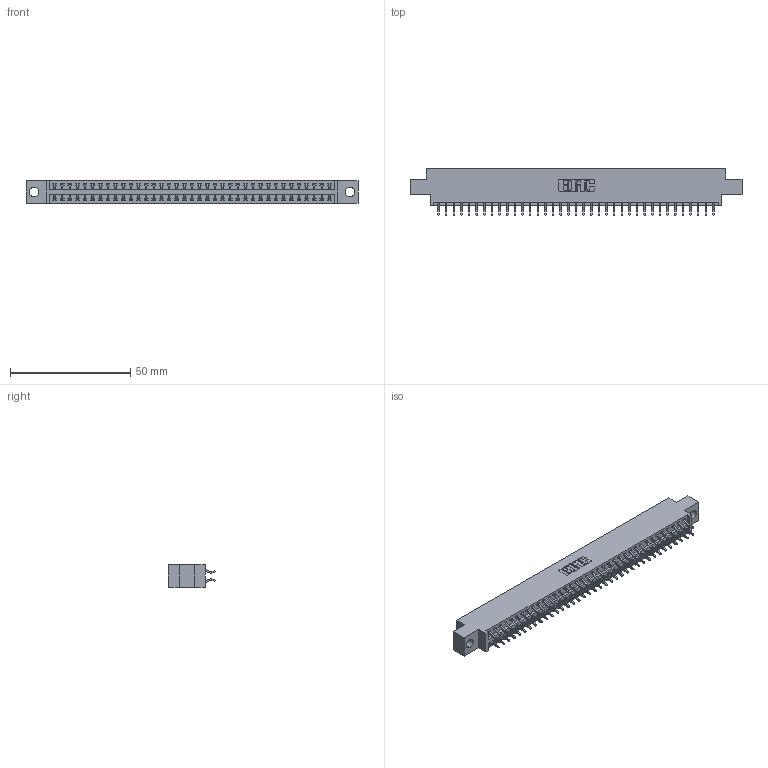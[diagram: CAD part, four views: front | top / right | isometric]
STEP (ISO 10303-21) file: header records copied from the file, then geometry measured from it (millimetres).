
FILE_DESCRIPTION (( 'STEP AP203' ), '1' );
FILE_NAME ('346-074-556-804.STEP', '2018-08-29T02:53:42', ( '' ), ( '' ), 'SwSTEP 2.0', 'SolidWorks 2016', '' );
FILE_SCHEMA (( 'CONFIG_CONTROL_DESIGN' ));
Length unit declared in the file: inch
Products named in the file (3): 346-074-556-804; 346 Part_0.170 Offset - 0.156 Dia-TH; 345-292-001_556 Tail
Assembly tree (75 placements, depth 2):
  346-074-556-804
    346 Part_0.170 Offset - 0.156 Dia-TH
    345-292-001_556 Tail  x74
Bounding box: 138.05 x 19.57 x 9.4 mm (x, y, z)
Volume: 13177.3 mm3; surface area: 17958.7 mm2
Topology: 75 solids, 75 shells, 4418 faces, 13143 edges, 8662 vertices
Faces by surface type: plane 2966, cylinder 1452
Entity records: 25175 total; most frequent: CARTESIAN_POINT 4172, ORIENTED_EDGE 4094, DIRECTION 3715, EDGE_CURVE 2047, VECTOR 1759, LINE 1759, VERTEX_POINT 1362, AXIS2_PLACEMENT_3D 978
